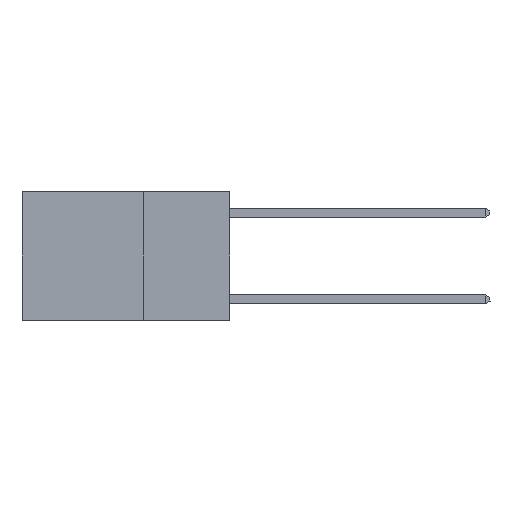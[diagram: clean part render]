
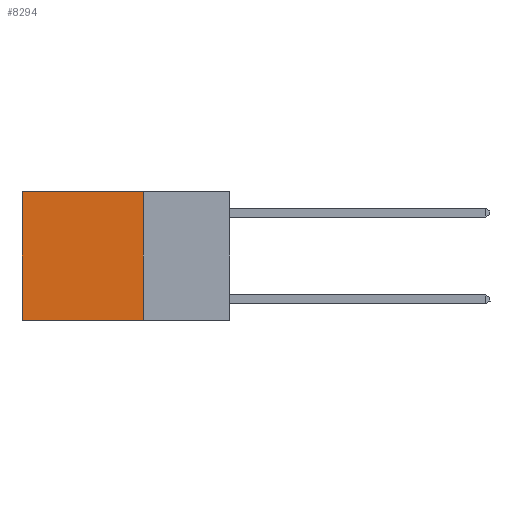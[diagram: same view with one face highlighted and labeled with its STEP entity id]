
A CAD part, left-side view. The second image highlights one B-rep face of the part: STEP entity #8294.
In plain terms, the highlighted planar face has unit normal (-1, 0, 0).
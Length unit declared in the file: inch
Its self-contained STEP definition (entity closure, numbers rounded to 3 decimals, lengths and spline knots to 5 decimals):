
#8 = DIRECTION ( 'NONE',  ( 0., 1., 0. ) ) ;
#178 = PLANE ( 'NONE',  #6420 ) ;
#518 = ORIENTED_EDGE ( 'NONE', *, *, #7367, .F. ) ;
#739 = ORIENTED_EDGE ( 'NONE', *, *, #8510, .T. ) ;
#1219 = DIRECTION ( 'NONE',  ( 0., 0., -1. ) ) ;
#1588 = CARTESIAN_POINT ( 'NONE',  ( 0.2625, 0.25, -0.37 ) ) ;
#2038 = VERTEX_POINT ( 'NONE', #5548 ) ;
#2343 = ORIENTED_EDGE ( 'NONE', *, *, #12825, .F. ) ;
#2565 = VECTOR ( 'NONE', #8, 39.37008 ) ;
#2604 = DIRECTION ( 'NONE',  ( 0., 1., 0. ) ) ;
#2739 = CARTESIAN_POINT ( 'NONE',  ( 0.2625, 0.6, -0.37 ) ) ;
#3128 = VECTOR ( 'NONE', #2604, 39.37008 ) ;
#3441 = VERTEX_POINT ( 'NONE', #5943 ) ;
#3450 = LINE ( 'NONE', #1588, #3128 ) ;
#3492 = CARTESIAN_POINT ( 'NONE',  ( 0.2625, 0.25, 0. ) ) ;
#3648 = LINE ( 'NONE', #5599, #6315 ) ;
#3863 = EDGE_CURVE ( 'NONE', #3441, #10512, #7694, .T. ) ;
#4836 = DIRECTION ( 'NONE',  ( 0., 0., -1. ) ) ;
#5218 = CARTESIAN_POINT ( 'NONE',  ( 0.2625, 0.25, 0. ) ) ;
#5548 = CARTESIAN_POINT ( 'NONE',  ( 0.2625, 0.25, -0.37 ) ) ;
#5599 = CARTESIAN_POINT ( 'NONE',  ( 0.2625, 0.25, 0. ) ) ;
#5623 = FACE_OUTER_BOUND ( 'NONE', #8656, .T. ) ;
#5943 = CARTESIAN_POINT ( 'NONE',  ( 0.2625, 0.25, 0. ) ) ;
#6002 = ORIENTED_EDGE ( 'NONE', *, *, #3863, .T. ) ;
#6207 = CARTESIAN_POINT ( 'NONE',  ( 0.2625, 0.6, 0. ) ) ;
#6315 = VECTOR ( 'NONE', #12551, 39.37008 ) ;
#6420 = AXIS2_PLACEMENT_3D ( 'NONE', #5218, #7321, #1219 ) ;
#7321 = DIRECTION ( 'NONE',  ( 1., 0., 0. ) ) ;
#7367 = EDGE_CURVE ( 'NONE', #3441, #2038, #3648, .T. ) ;
#7694 = LINE ( 'NONE', #3492, #2565 ) ;
#8294 = ADVANCED_FACE ( 'NONE', ( #5623 ), #178, .F. ) ;
#8510 = EDGE_CURVE ( 'NONE', #10512, #10127, #9964, .T. ) ;
#8656 = EDGE_LOOP ( 'NONE', ( #739, #2343, #518, #6002 ) ) ;
#9964 = LINE ( 'NONE', #10876, #12465 ) ;
#10127 = VERTEX_POINT ( 'NONE', #2739 ) ;
#10512 = VERTEX_POINT ( 'NONE', #6207 ) ;
#10876 = CARTESIAN_POINT ( 'NONE',  ( 0.2625, 0.6, 0. ) ) ;
#12465 = VECTOR ( 'NONE', #4836, 39.37008 ) ;
#12551 = DIRECTION ( 'NONE',  ( 0., 0., -1. ) ) ;
#12825 = EDGE_CURVE ( 'NONE', #2038, #10127, #3450, .T. ) ;
